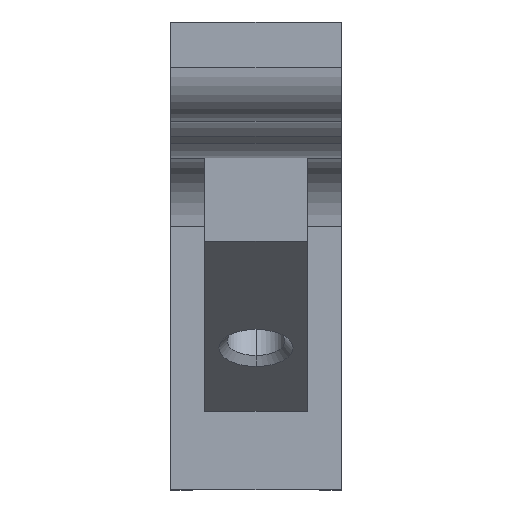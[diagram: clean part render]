
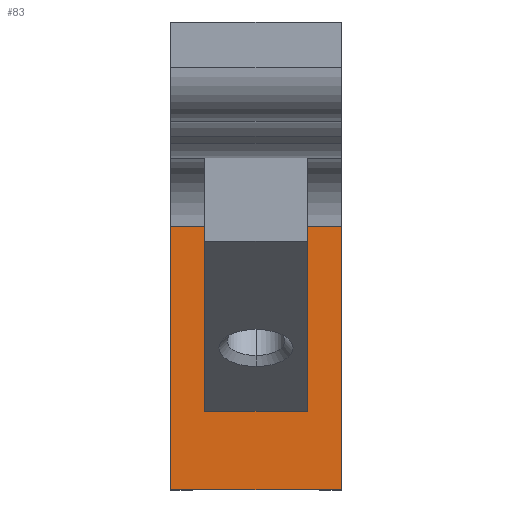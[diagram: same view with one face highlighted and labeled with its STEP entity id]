
A CAD part, top view. The second image highlights one B-rep face of the part: STEP entity #83.
In plain terms, the highlighted planar face has unit normal (0, 0, 1).
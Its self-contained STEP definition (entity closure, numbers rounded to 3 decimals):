
#17 = DIRECTION ( 'NONE',  ( -1., 0., 0. ) ) ;
#31 = ORIENTED_EDGE ( 'NONE', *, *, #460, .T. ) ;
#83 = ADVANCED_FACE ( 'NONE', ( #805 ), #1571, .T. ) ;
#177 = ORIENTED_EDGE ( 'NONE', *, *, #1295, .F. ) ;
#187 = CARTESIAN_POINT ( 'NONE',  ( 7.938, 24.581, 10.16 ) ) ;
#194 = LINE ( 'NONE', #1539, #1970 ) ;
#203 = CARTESIAN_POINT ( 'NONE',  ( -7.938, 24.581, 10.16 ) ) ;
#244 = VECTOR ( 'NONE', #306, 1000. ) ;
#303 = ORIENTED_EDGE ( 'NONE', *, *, #1355, .F. ) ;
#306 = DIRECTION ( 'NONE',  ( 0., 1., 0. ) ) ;
#381 = CARTESIAN_POINT ( 'NONE',  ( 7.938, 0., 10.16 ) ) ;
#394 = VERTEX_POINT ( 'NONE', #720 ) ;
#395 = CARTESIAN_POINT ( 'NONE',  ( 4.762, 24.581, 10.16 ) ) ;
#401 = LINE ( 'NONE', #795, #2297 ) ;
#402 = CARTESIAN_POINT ( 'NONE',  ( -4.762, 7.315, 10.16 ) ) ;
#415 = EDGE_CURVE ( 'NONE', #2237, #2346, #1551, .T. ) ;
#428 = EDGE_CURVE ( 'NONE', #1976, #2237, #194, .T. ) ;
#460 = EDGE_CURVE ( 'NONE', #1015, #2027, #1738, .T. ) ;
#475 = CARTESIAN_POINT ( 'NONE',  ( -7.938, 0., 10.16 ) ) ;
#485 = VECTOR ( 'NONE', #2347, 1000. ) ;
#492 = ORIENTED_EDGE ( 'NONE', *, *, #428, .F. ) ;
#510 = DIRECTION ( 'NONE',  ( 0., -1., 0. ) ) ;
#569 = AXIS2_PLACEMENT_3D ( 'NONE', #1730, #2079, #2157 ) ;
#583 = VECTOR ( 'NONE', #1339, 1000. ) ;
#665 = ORIENTED_EDGE ( 'NONE', *, *, #1620, .T. ) ;
#720 = CARTESIAN_POINT ( 'NONE',  ( -4.762, 7.315, 10.16 ) ) ;
#739 = DIRECTION ( 'NONE',  ( -1., 0., 0. ) ) ;
#740 = CARTESIAN_POINT ( 'NONE',  ( -4.762, 24.581, 10.16 ) ) ;
#742 = ORIENTED_EDGE ( 'NONE', *, *, #2339, .F. ) ;
#747 = DIRECTION ( 'NONE',  ( -1., 0., 0. ) ) ;
#795 = CARTESIAN_POINT ( 'NONE',  ( 8.763, 0., 10.16 ) ) ;
#805 = FACE_OUTER_BOUND ( 'NONE', #2156, .T. ) ;
#808 = VERTEX_POINT ( 'NONE', #381 ) ;
#924 = LINE ( 'NONE', #1701, #1176 ) ;
#976 = DIRECTION ( 'NONE',  ( 0., 1., 0. ) ) ;
#1015 = VERTEX_POINT ( 'NONE', #740 ) ;
#1031 = EDGE_CURVE ( 'NONE', #394, #1015, #1759, .T. ) ;
#1176 = VECTOR ( 'NONE', #747, 1000. ) ;
#1229 = VECTOR ( 'NONE', #17, 1000. ) ;
#1261 = LINE ( 'NONE', #475, #244 ) ;
#1295 = EDGE_CURVE ( 'NONE', #1624, #2027, #1261, .T. ) ;
#1339 = DIRECTION ( 'NONE',  ( 0., 1., 0. ) ) ;
#1355 = EDGE_CURVE ( 'NONE', #2346, #808, #1846, .T. ) ;
#1449 = VECTOR ( 'NONE', #510, 1000. ) ;
#1490 = CARTESIAN_POINT ( 'NONE',  ( 7.938, 24.581, 10.16 ) ) ;
#1539 = CARTESIAN_POINT ( 'NONE',  ( 4.762, 7.315, 10.16 ) ) ;
#1551 = LINE ( 'NONE', #395, #485 ) ;
#1571 = PLANE ( 'NONE',  #569 ) ;
#1620 = EDGE_CURVE ( 'NONE', #1976, #394, #924, .T. ) ;
#1624 = VERTEX_POINT ( 'NONE', #2479 ) ;
#1679 = CARTESIAN_POINT ( 'NONE',  ( 4.762, 24.581, 10.16 ) ) ;
#1701 = CARTESIAN_POINT ( 'NONE',  ( 8.763, 7.315, 10.16 ) ) ;
#1730 = CARTESIAN_POINT ( 'NONE',  ( 8.763, 0., 10.16 ) ) ;
#1738 = LINE ( 'NONE', #1940, #1229 ) ;
#1759 = LINE ( 'NONE', #402, #583 ) ;
#1846 = LINE ( 'NONE', #1490, #1449 ) ;
#1940 = CARTESIAN_POINT ( 'NONE',  ( -4.762, 24.581, 10.16 ) ) ;
#1970 = VECTOR ( 'NONE', #976, 1000. ) ;
#1976 = VERTEX_POINT ( 'NONE', #2325 ) ;
#2027 = VERTEX_POINT ( 'NONE', #203 ) ;
#2039 = ORIENTED_EDGE ( 'NONE', *, *, #1031, .T. ) ;
#2079 = DIRECTION ( 'NONE',  ( 0., 0., 1. ) ) ;
#2156 = EDGE_LOOP ( 'NONE', ( #742, #303, #2477, #492, #665, #2039, #31, #177 ) ) ;
#2157 = DIRECTION ( 'NONE',  ( 1., 0., 0. ) ) ;
#2237 = VERTEX_POINT ( 'NONE', #1679 ) ;
#2297 = VECTOR ( 'NONE', #739, 1000. ) ;
#2325 = CARTESIAN_POINT ( 'NONE',  ( 4.762, 7.315, 10.16 ) ) ;
#2339 = EDGE_CURVE ( 'NONE', #808, #1624, #401, .T. ) ;
#2346 = VERTEX_POINT ( 'NONE', #187 ) ;
#2347 = DIRECTION ( 'NONE',  ( 1., 0., 0. ) ) ;
#2477 = ORIENTED_EDGE ( 'NONE', *, *, #415, .F. ) ;
#2479 = CARTESIAN_POINT ( 'NONE',  ( -7.938, 0., 10.16 ) ) ;
